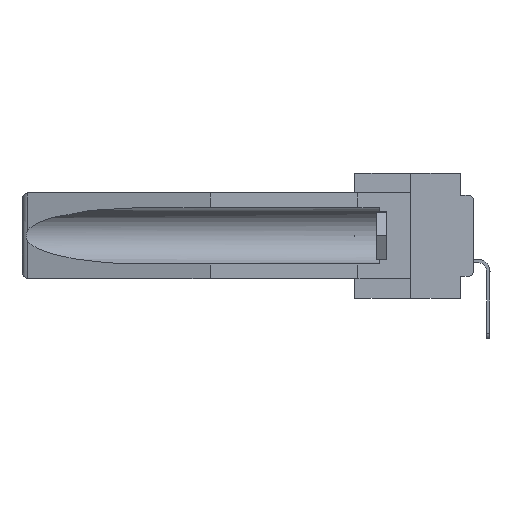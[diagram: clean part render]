
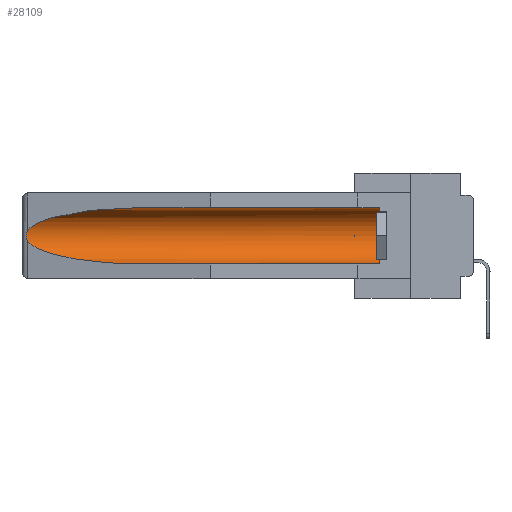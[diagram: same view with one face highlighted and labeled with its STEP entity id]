
A CAD part, left-side view. The second image highlights one B-rep face of the part: STEP entity #28109.
In plain terms, the highlighted cylindrical face has radius 2.857 mm (diameter 5.715 mm), a partial arc.
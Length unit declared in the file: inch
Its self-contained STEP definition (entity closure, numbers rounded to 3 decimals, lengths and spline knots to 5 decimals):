
#334 = LINE ( 'NONE', #12230, #28276 ) ;
#349 = CARTESIAN_POINT ( 'NONE',  ( 0.26537, 1.52718, -0.14972 ) ) ;
#502 = DIRECTION ( 'NONE',  ( 0., -1., 0. ) ) ;
#2344 = ORIENTED_EDGE ( 'NONE', *, *, #28087, .T. ) ;
#2685 = DIRECTION ( 'NONE',  ( 0., 1., 0. ) ) ;
#2762 = CIRCLE ( 'NONE', #30150, 0.1125 ) ;
#2885 = CARTESIAN_POINT ( 'NONE',  ( 0.155, 0.126, -0.059 ) ) ;
#3301 = ORIENTED_EDGE ( 'NONE', *, *, #29929, .T. ) ;
#3690 = VERTEX_POINT ( 'NONE', #5359 ) ;
#4006 = EDGE_LOOP ( 'NONE', ( #2344, #3301, #32407, #8453, #4131, #23389 ) ) ;
#4131 = ORIENTED_EDGE ( 'NONE', *, *, #23647, .T. ) ;
#5247 = CARTESIAN_POINT ( 'NONE',  ( 0.26537, 1.52718, -0.14972 ) ) ;
#5277 =( BOUNDED_CURVE ( )  B_SPLINE_CURVE ( 3, ( #27079, #29616, #24167, #349 ),
 .UNSPECIFIED., .F., .F. ) 
 B_SPLINE_CURVE_WITH_KNOTS ( ( 4, 4 ),
 ( 4.71239, 6.08839 ),
 .UNSPECIFIED. ) 
 CURVE ( )  GEOMETRIC_REPRESENTATION_ITEM ( )  RATIONAL_B_SPLINE_CURVE ( ( 1., 0.848, 0.848, 1. ) ) 
 REPRESENTATION_ITEM ( '' )  );
#5359 = CARTESIAN_POINT ( 'NONE',  ( 0.155, 1.07973, -0.284 ) ) ;
#6396 = CYLINDRICAL_SURFACE ( 'NONE', #24897, 0.1125 ) ;
#8453 = ORIENTED_EDGE ( 'NONE', *, *, #12451, .F. ) ;
#8833 = VERTEX_POINT ( 'NONE', #5247 ) ;
#8864 = VERTEX_POINT ( 'NONE', #2885 ) ;
#8865 = B_SPLINE_CURVE_WITH_KNOTS ( 'NONE', 3,
 ( #21134, #11967, #38511, #17456, #11779, #23694, #14902, #18013, #20575, #15090 ),
 .UNSPECIFIED., .F., .F.,
 ( 4, 2, 2, 2, 4 ),
 ( 0., 0.00029, 0.00058, 0.00087, 0.00117 ),
 .UNSPECIFIED. ) ;
#11779 = CARTESIAN_POINT ( 'NONE',  ( 0.2675, 1.53308, -0.16763 ) ) ;
#11878 = CARTESIAN_POINT ( 'NONE',  ( 0.21114, 1.30732, -0.284 ) ) ;
#11967 = CARTESIAN_POINT ( 'NONE',  ( 0.26597, 1.52961, -0.15275 ) ) ;
#12230 = CARTESIAN_POINT ( 'NONE',  ( 0.155, -0.30754, -0.284 ) ) ;
#12451 = EDGE_CURVE ( 'NONE', #25605, #3690, #334, .T. ) ;
#13512 = CARTESIAN_POINT ( 'NONE',  ( 0.155, -0.30754, -0.059 ) ) ;
#14616 = DIRECTION ( 'NONE',  ( 0., 1., 0. ) ) ;
#14902 = CARTESIAN_POINT ( 'NONE',  ( 0.2673, 1.53269, -0.17917 ) ) ;
#15090 = CARTESIAN_POINT ( 'NONE',  ( 0.26537, 1.52718, -0.19328 ) ) ;
#15175 = FACE_OUTER_BOUND ( 'NONE', #4006, .T. ) ;
#15343 = CARTESIAN_POINT ( 'NONE',  ( 0.26537, 1.52718, -0.19328 ) ) ;
#16828 = LINE ( 'NONE', #13512, #20113 ) ;
#17456 = CARTESIAN_POINT ( 'NONE',  ( 0.2673, 1.5327, -0.16383 ) ) ;
#17733 = CARTESIAN_POINT ( 'NONE',  ( 0.155, -0.30754, -0.1715 ) ) ;
#18013 = CARTESIAN_POINT ( 'NONE',  ( 0.26655, 1.53094, -0.18657 ) ) ;
#20113 = VECTOR ( 'NONE', #25811, 39.37008 ) ;
#20575 = CARTESIAN_POINT ( 'NONE',  ( 0.26597, 1.5296, -0.19026 ) ) ;
#20723 = VERTEX_POINT ( 'NONE', #29103 ) ;
#20810 = EDGE_CURVE ( 'NONE', #8864, #20723, #16828, .T. ) ;
#21134 = CARTESIAN_POINT ( 'NONE',  ( 0.26537, 1.52718, -0.14972 ) ) ;
#21757 = CARTESIAN_POINT ( 'NONE',  ( 0.155, 0.126, -0.1715 ) ) ;
#21954 = DIRECTION ( 'NONE',  ( 0., 0., 1. ) ) ;
#22692 = EDGE_CURVE ( 'NONE', #34059, #3690, #32943, .T. ) ;
#23389 = ORIENTED_EDGE ( 'NONE', *, *, #20810, .T. ) ;
#23647 = EDGE_CURVE ( 'NONE', #25605, #8864, #2762, .T. ) ;
#23694 = CARTESIAN_POINT ( 'NONE',  ( 0.2675, 1.53308, -0.17534 ) ) ;
#23793 = CARTESIAN_POINT ( 'NONE',  ( 0.26537, 1.52718, -0.19328 ) ) ;
#24167 = CARTESIAN_POINT ( 'NONE',  ( 0.25451, 1.48313, -0.09465 ) ) ;
#24897 = AXIS2_PLACEMENT_3D ( 'NONE', #17733, #14616, #30178 ) ;
#25605 = VERTEX_POINT ( 'NONE', #26194 ) ;
#25811 = DIRECTION ( 'NONE',  ( 0., 1., 0. ) ) ;
#26194 = CARTESIAN_POINT ( 'NONE',  ( 0.155, 0.126, -0.284 ) ) ;
#26537 = CARTESIAN_POINT ( 'NONE',  ( 0.25451, 1.48313, -0.24835 ) ) ;
#27079 = CARTESIAN_POINT ( 'NONE',  ( 0.155, 1.07973, -0.059 ) ) ;
#28087 = EDGE_CURVE ( 'NONE', #20723, #8833, #5277, .T. ) ;
#28109 = ADVANCED_FACE ( 'NONE', ( #15175 ), #6396, .F. ) ;
#28276 = VECTOR ( 'NONE', #2685, 39.37008 ) ;
#29103 = CARTESIAN_POINT ( 'NONE',  ( 0.155, 1.07973, -0.059 ) ) ;
#29616 = CARTESIAN_POINT ( 'NONE',  ( 0.21114, 1.30732, -0.059 ) ) ;
#29929 = EDGE_CURVE ( 'NONE', #8833, #34059, #8865, .T. ) ;
#30150 = AXIS2_PLACEMENT_3D ( 'NONE', #21757, #502, #21954 ) ;
#30178 = DIRECTION ( 'NONE',  ( 0., 0., 1. ) ) ;
#32407 = ORIENTED_EDGE ( 'NONE', *, *, #22692, .T. ) ;
#32943 =( BOUNDED_CURVE ( )  B_SPLINE_CURVE ( 3, ( #23793, #26537, #11878, #32946 ),
 .UNSPECIFIED., .F., .F. ) 
 B_SPLINE_CURVE_WITH_KNOTS ( ( 4, 4 ),
 ( 0.1948, 1.5708 ),
 .UNSPECIFIED. ) 
 CURVE ( )  GEOMETRIC_REPRESENTATION_ITEM ( )  RATIONAL_B_SPLINE_CURVE ( ( 1., 0.848, 0.848, 1. ) ) 
 REPRESENTATION_ITEM ( '' )  );
#32946 = CARTESIAN_POINT ( 'NONE',  ( 0.155, 1.07973, -0.284 ) ) ;
#34059 = VERTEX_POINT ( 'NONE', #15343 ) ;
#38511 = CARTESIAN_POINT ( 'NONE',  ( 0.26654, 1.53092, -0.15636 ) ) ;
